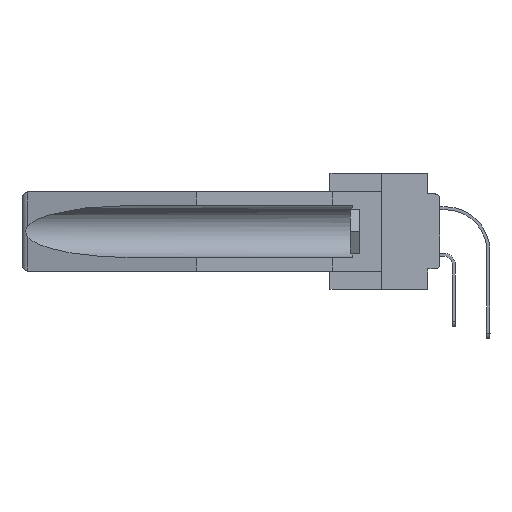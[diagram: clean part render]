
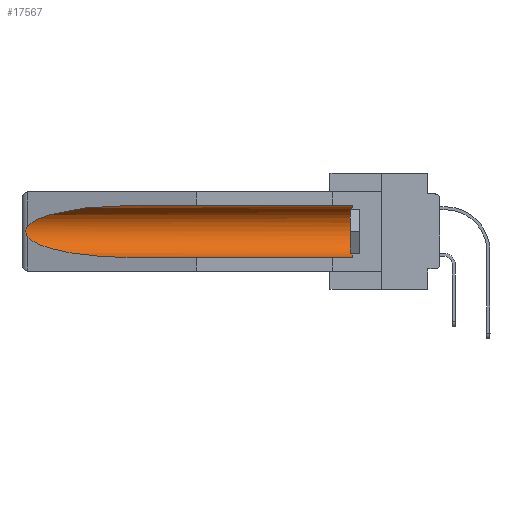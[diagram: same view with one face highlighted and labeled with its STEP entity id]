
A CAD part, left-side view. The second image highlights one B-rep face of the part: STEP entity #17567.
In plain terms, the highlighted cylindrical face has radius 2.857 mm (diameter 5.715 mm), a partial arc.
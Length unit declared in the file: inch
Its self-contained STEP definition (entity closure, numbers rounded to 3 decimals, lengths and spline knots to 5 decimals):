
#307 = CARTESIAN_POINT ( 'NONE',  ( 0.26537, 1.52718, -0.14972 ) ) ;
#964 = CARTESIAN_POINT ( 'NONE',  ( 0.26537, 1.52718, -0.14972 ) ) ;
#1360 = EDGE_CURVE ( 'NONE', #19872, #39695, #28195, .T. ) ;
#1523 = DIRECTION ( 'NONE',  ( 0., 1., 0. ) ) ;
#2009 = CARTESIAN_POINT ( 'NONE',  ( 0.26597, 1.52961, -0.15275 ) ) ;
#3636 = DIRECTION ( 'NONE',  ( 0., -1., 0. ) ) ;
#3822 = DIRECTION ( 'NONE',  ( 0., 0., 1. ) ) ;
#4523 = B_SPLINE_CURVE_WITH_KNOTS ( 'NONE', 3,
 ( #39925, #2009, #5093, #33600, #24159, #36659, #29735, #20689, #27250, #20271 ),
 .UNSPECIFIED., .F., .F.,
 ( 4, 2, 2, 2, 4 ),
 ( 0., 0.00029, 0.00058, 0.00087, 0.00117 ),
 .UNSPECIFIED. ) ;
#5093 = CARTESIAN_POINT ( 'NONE',  ( 0.26654, 1.53092, -0.15636 ) ) ;
#5371 = EDGE_CURVE ( 'NONE', #39695, #17530, #35968, .T. ) ;
#6440 = CARTESIAN_POINT ( 'NONE',  ( 0.155, 1.07973, -0.059 ) ) ;
#6700 = CARTESIAN_POINT ( 'NONE',  ( 0.155, 1.07973, -0.284 ) ) ;
#7199 = VERTEX_POINT ( 'NONE', #35118 ) ;
#7899 = DIRECTION ( 'NONE',  ( 0., 0., 1. ) ) ;
#8517 = VERTEX_POINT ( 'NONE', #35264 ) ;
#9720 = CARTESIAN_POINT ( 'NONE',  ( 0.155, 1.07973, -0.059 ) ) ;
#9771 = CARTESIAN_POINT ( 'NONE',  ( 0.26537, 1.52718, -0.19328 ) ) ;
#9878 = ORIENTED_EDGE ( 'NONE', *, *, #25715, .T. ) ;
#10807 = DIRECTION ( 'NONE',  ( 0., 1., 0. ) ) ;
#11033 = ORIENTED_EDGE ( 'NONE', *, *, #26404, .F. ) ;
#11227 = VERTEX_POINT ( 'NONE', #38767 ) ;
#13020 = ORIENTED_EDGE ( 'NONE', *, *, #5371, .T. ) ;
#13653 = CYLINDRICAL_SURFACE ( 'NONE', #28925, 0.1125 ) ;
#16782 = CARTESIAN_POINT ( 'NONE',  ( 0.155, 0.126, -0.059 ) ) ;
#17436 = EDGE_CURVE ( 'NONE', #7199, #8517, #38594, .T. ) ;
#17530 = VERTEX_POINT ( 'NONE', #964 ) ;
#17567 = ADVANCED_FACE ( 'NONE', ( #38878 ), #13653, .F. ) ;
#18139 = ORIENTED_EDGE ( 'NONE', *, *, #34617, .T. ) ;
#19430 = AXIS2_PLACEMENT_3D ( 'NONE', #28452, #3636, #3822 ) ;
#19872 = VERTEX_POINT ( 'NONE', #16782 ) ;
#20009 = EDGE_LOOP ( 'NONE', ( #13020, #18139, #31148, #11033, #9878, #36344 ) ) ;
#20271 = CARTESIAN_POINT ( 'NONE',  ( 0.26537, 1.52718, -0.19328 ) ) ;
#20689 = CARTESIAN_POINT ( 'NONE',  ( 0.26655, 1.53094, -0.18657 ) ) ;
#21836 = CARTESIAN_POINT ( 'NONE',  ( 0.25451, 1.48313, -0.09465 ) ) ;
#22267 = CARTESIAN_POINT ( 'NONE',  ( 0.25451, 1.48313, -0.24835 ) ) ;
#24159 = CARTESIAN_POINT ( 'NONE',  ( 0.2675, 1.53308, -0.16763 ) ) ;
#25131 = CARTESIAN_POINT ( 'NONE',  ( 0.155, -0.30754, -0.059 ) ) ;
#25715 = EDGE_CURVE ( 'NONE', #11227, #19872, #33169, .T. ) ;
#26404 = EDGE_CURVE ( 'NONE', #11227, #8517, #32683, .T. ) ;
#27250 = CARTESIAN_POINT ( 'NONE',  ( 0.26597, 1.5296, -0.19026 ) ) ;
#27947 = VECTOR ( 'NONE', #1523, 39.37008 ) ;
#28195 = LINE ( 'NONE', #25131, #36246 ) ;
#28452 = CARTESIAN_POINT ( 'NONE',  ( 0.155, 0.126, -0.1715 ) ) ;
#28925 = AXIS2_PLACEMENT_3D ( 'NONE', #39075, #10807, #7899 ) ;
#29608 = CARTESIAN_POINT ( 'NONE',  ( 0.155, -0.30754, -0.284 ) ) ;
#29735 = CARTESIAN_POINT ( 'NONE',  ( 0.2673, 1.53269, -0.17917 ) ) ;
#31148 = ORIENTED_EDGE ( 'NONE', *, *, #17436, .T. ) ;
#31478 = CARTESIAN_POINT ( 'NONE',  ( 0.21114, 1.30732, -0.059 ) ) ;
#32683 = LINE ( 'NONE', #29608, #27947 ) ;
#33169 = CIRCLE ( 'NONE', #19430, 0.1125 ) ;
#33600 = CARTESIAN_POINT ( 'NONE',  ( 0.2673, 1.5327, -0.16383 ) ) ;
#34617 = EDGE_CURVE ( 'NONE', #17530, #7199, #4523, .T. ) ;
#34794 = CARTESIAN_POINT ( 'NONE',  ( 0.21114, 1.30732, -0.284 ) ) ;
#35118 = CARTESIAN_POINT ( 'NONE',  ( 0.26537, 1.52718, -0.19328 ) ) ;
#35264 = CARTESIAN_POINT ( 'NONE',  ( 0.155, 1.07973, -0.284 ) ) ;
#35968 =( BOUNDED_CURVE ( )  B_SPLINE_CURVE ( 3, ( #6440, #31478, #21836, #307 ),
 .UNSPECIFIED., .F., .F. ) 
 B_SPLINE_CURVE_WITH_KNOTS ( ( 4, 4 ),
 ( 4.71239, 6.08839 ),
 .UNSPECIFIED. ) 
 CURVE ( )  GEOMETRIC_REPRESENTATION_ITEM ( )  RATIONAL_B_SPLINE_CURVE ( ( 1., 0.848, 0.848, 1. ) ) 
 REPRESENTATION_ITEM ( '' )  );
#36246 = VECTOR ( 'NONE', #37625, 39.37008 ) ;
#36344 = ORIENTED_EDGE ( 'NONE', *, *, #1360, .T. ) ;
#36659 = CARTESIAN_POINT ( 'NONE',  ( 0.2675, 1.53308, -0.17534 ) ) ;
#37625 = DIRECTION ( 'NONE',  ( 0., 1., 0. ) ) ;
#38594 =( BOUNDED_CURVE ( )  B_SPLINE_CURVE ( 3, ( #9771, #22267, #34794, #6700 ),
 .UNSPECIFIED., .F., .F. ) 
 B_SPLINE_CURVE_WITH_KNOTS ( ( 4, 4 ),
 ( 0.1948, 1.5708 ),
 .UNSPECIFIED. ) 
 CURVE ( )  GEOMETRIC_REPRESENTATION_ITEM ( )  RATIONAL_B_SPLINE_CURVE ( ( 1., 0.848, 0.848, 1. ) ) 
 REPRESENTATION_ITEM ( '' )  );
#38767 = CARTESIAN_POINT ( 'NONE',  ( 0.155, 0.126, -0.284 ) ) ;
#38878 = FACE_OUTER_BOUND ( 'NONE', #20009, .T. ) ;
#39075 = CARTESIAN_POINT ( 'NONE',  ( 0.155, -0.30754, -0.1715 ) ) ;
#39695 = VERTEX_POINT ( 'NONE', #9720 ) ;
#39925 = CARTESIAN_POINT ( 'NONE',  ( 0.26537, 1.52718, -0.14972 ) ) ;
